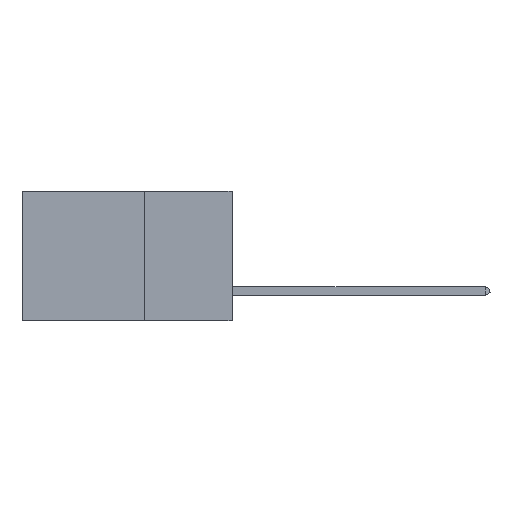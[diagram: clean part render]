
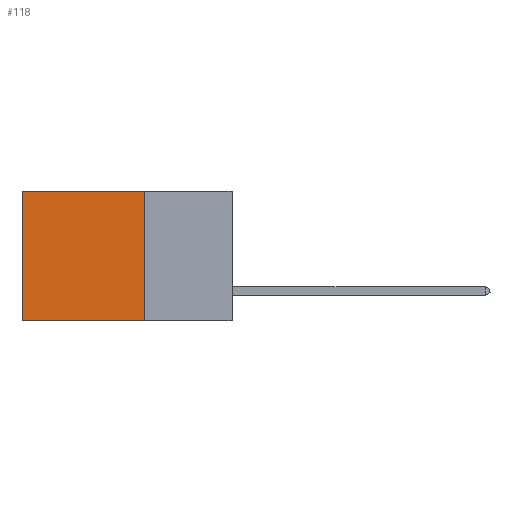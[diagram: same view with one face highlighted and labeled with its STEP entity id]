
A CAD part, left-side view. The second image highlights one B-rep face of the part: STEP entity #118.
In plain terms, the highlighted planar face has unit normal (-1, 0, 0).
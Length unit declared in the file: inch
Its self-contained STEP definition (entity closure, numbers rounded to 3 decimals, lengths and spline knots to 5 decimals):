
#118 = ADVANCED_FACE ( 'NONE', ( #5325 ), #14474, .F. ) ;
#354 = CARTESIAN_POINT ( 'NONE',  ( 0.2875, 0.25, 0. ) ) ;
#2330 = CARTESIAN_POINT ( 'NONE',  ( 0.2875, 0.25, 0. ) ) ;
#3504 = DIRECTION ( 'NONE',  ( 1., 0., 0. ) ) ;
#5325 = FACE_OUTER_BOUND ( 'NONE', #35823, .T. ) ;
#5816 = VECTOR ( 'NONE', #19201, 39.37008 ) ;
#6105 = VERTEX_POINT ( 'NONE', #27224 ) ;
#8444 = CARTESIAN_POINT ( 'NONE',  ( 0.2875, 0.25, -0.37 ) ) ;
#8550 = ORIENTED_EDGE ( 'NONE', *, *, #35099, .T. ) ;
#9069 = DIRECTION ( 'NONE',  ( 0., 0., -1. ) ) ;
#9389 = DIRECTION ( 'NONE',  ( 0., 1., 0. ) ) ;
#10794 = VERTEX_POINT ( 'NONE', #37710 ) ;
#13490 = CARTESIAN_POINT ( 'NONE',  ( 0.2875, 0.25, 0. ) ) ;
#14474 = PLANE ( 'NONE',  #24169 ) ;
#14519 = EDGE_CURVE ( 'NONE', #10794, #28510, #21402, .T. ) ;
#14520 = EDGE_CURVE ( 'NONE', #6105, #28510, #22008, .T. ) ;
#15351 = VECTOR ( 'NONE', #9069, 39.37008 ) ;
#16496 = CARTESIAN_POINT ( 'NONE',  ( 0.2875, 0.25, 0. ) ) ;
#16678 = LINE ( 'NONE', #2330, #41740 ) ;
#19201 = DIRECTION ( 'NONE',  ( 0., 1., 0. ) ) ;
#19814 = CARTESIAN_POINT ( 'NONE',  ( 0.2875, 0.6, 0. ) ) ;
#21402 = LINE ( 'NONE', #19814, #15351 ) ;
#22008 = LINE ( 'NONE', #8444, #5816 ) ;
#24169 = AXIS2_PLACEMENT_3D ( 'NONE', #354, #3504, #28461 ) ;
#25463 = EDGE_CURVE ( 'NONE', #34518, #6105, #34819, .T. ) ;
#27224 = CARTESIAN_POINT ( 'NONE',  ( 0.2875, 0.25, -0.37 ) ) ;
#28209 = ORIENTED_EDGE ( 'NONE', *, *, #25463, .F. ) ;
#28461 = DIRECTION ( 'NONE',  ( 0., 0., -1. ) ) ;
#28510 = VERTEX_POINT ( 'NONE', #39587 ) ;
#30955 = ORIENTED_EDGE ( 'NONE', *, *, #14519, .T. ) ;
#34518 = VERTEX_POINT ( 'NONE', #13490 ) ;
#34819 = LINE ( 'NONE', #16496, #43165 ) ;
#35099 = EDGE_CURVE ( 'NONE', #34518, #10794, #16678, .T. ) ;
#35823 = EDGE_LOOP ( 'NONE', ( #30955, #43968, #28209, #8550 ) ) ;
#37710 = CARTESIAN_POINT ( 'NONE',  ( 0.2875, 0.6, 0. ) ) ;
#39587 = CARTESIAN_POINT ( 'NONE',  ( 0.2875, 0.6, -0.37 ) ) ;
#41740 = VECTOR ( 'NONE', #9389, 39.37008 ) ;
#43165 = VECTOR ( 'NONE', #45438, 39.37008 ) ;
#43968 = ORIENTED_EDGE ( 'NONE', *, *, #14520, .F. ) ;
#45438 = DIRECTION ( 'NONE',  ( 0., 0., -1. ) ) ;
